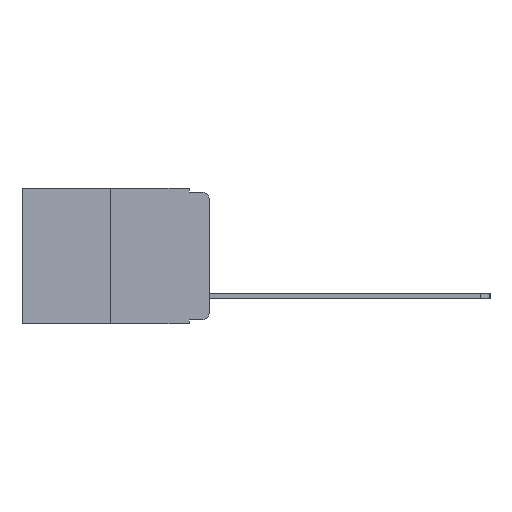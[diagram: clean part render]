
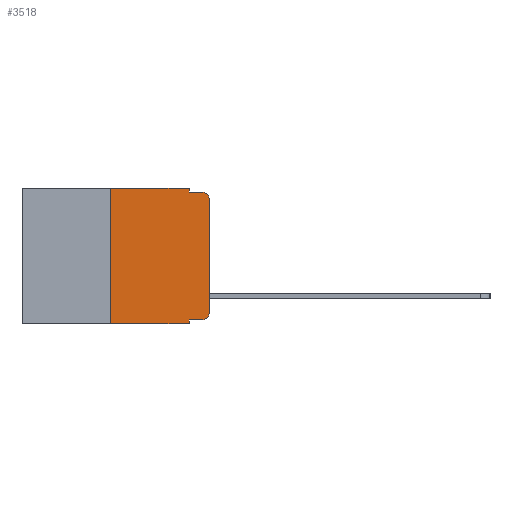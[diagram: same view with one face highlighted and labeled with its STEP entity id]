
A CAD part, left-side view. The second image highlights one B-rep face of the part: STEP entity #3518.
In plain terms, the highlighted planar face has unit normal (-1, 0, 0).
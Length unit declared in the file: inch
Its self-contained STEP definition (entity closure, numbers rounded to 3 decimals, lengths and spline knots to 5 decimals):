
#81 = CARTESIAN_POINT ( 'NONE',  ( 0., 0.473, 0. ) ) ;
#176 = ORIENTED_EDGE ( 'NONE', *, *, #246, .F. ) ;
#246 = EDGE_CURVE ( 'NONE', #16727, #5593, #1035, .T. ) ;
#524 = CARTESIAN_POINT ( 'NONE',  ( 0., 0.25, -0.343 ) ) ;
#882 = DIRECTION ( 'NONE',  ( 0., 0., -1. ) ) ;
#1035 = LINE ( 'NONE', #6684, #17609 ) ;
#1259 = ORIENTED_EDGE ( 'NONE', *, *, #16861, .T. ) ;
#1407 = EDGE_CURVE ( 'NONE', #2608, #8462, #6158, .T. ) ;
#1764 = DIRECTION ( 'NONE',  ( 0., 0., 1. ) ) ;
#1791 = ORIENTED_EDGE ( 'NONE', *, *, #15820, .T. ) ;
#1951 = CARTESIAN_POINT ( 'NONE',  ( 0., 0.02, -0.03 ) ) ;
#1986 = EDGE_CURVE ( 'NONE', #16727, #6013, #12176, .T. ) ;
#1997 = FACE_OUTER_BOUND ( 'NONE', #14314, .T. ) ;
#2320 = CARTESIAN_POINT ( 'NONE',  ( 0., 0.051, 0. ) ) ;
#2608 = VERTEX_POINT ( 'NONE', #2320 ) ;
#3518 = ADVANCED_FACE ( 'NONE', ( #1997 ), #7700, .F. ) ;
#3572 = ORIENTED_EDGE ( 'NONE', *, *, #1407, .F. ) ;
#3592 = DIRECTION ( 'NONE',  ( 0., 0., -1. ) ) ;
#4087 = ORIENTED_EDGE ( 'NONE', *, *, #7369, .F. ) ;
#4535 = DIRECTION ( 'NONE',  ( 1., 0., 0. ) ) ;
#4538 = CARTESIAN_POINT ( 'NONE',  ( 0., 0.051, -0.01 ) ) ;
#4600 = ORIENTED_EDGE ( 'NONE', *, *, #1986, .T. ) ;
#4641 = LINE ( 'NONE', #10688, #7469 ) ;
#4719 = EDGE_CURVE ( 'NONE', #8462, #19541, #13377, .T. ) ;
#4945 = VERTEX_POINT ( 'NONE', #5145 ) ;
#5006 = CARTESIAN_POINT ( 'NONE',  ( 0., 0., 0. ) ) ;
#5089 = DIRECTION ( 'NONE',  ( 0., 0., -1. ) ) ;
#5116 = CARTESIAN_POINT ( 'NONE',  ( 0., 0., -0.313 ) ) ;
#5145 = CARTESIAN_POINT ( 'NONE',  ( 0., 0., -0.03 ) ) ;
#5188 = CARTESIAN_POINT ( 'NONE',  ( 0., 0.25, 0. ) ) ;
#5298 = CARTESIAN_POINT ( 'NONE',  ( 0., 0.02, -0.01 ) ) ;
#5566 = VERTEX_POINT ( 'NONE', #5116 ) ;
#5593 = VERTEX_POINT ( 'NONE', #5188 ) ;
#5675 = CARTESIAN_POINT ( 'NONE',  ( 0., 0.051, -0.333 ) ) ;
#6013 = VERTEX_POINT ( 'NONE', #10946 ) ;
#6158 = LINE ( 'NONE', #6173, #18783 ) ;
#6173 = CARTESIAN_POINT ( 'NONE',  ( 0., 0.051, 0. ) ) ;
#6302 = CARTESIAN_POINT ( 'NONE',  ( 0., 0.02, -0.313 ) ) ;
#6607 = DIRECTION ( 'NONE',  ( 0., -1., 0. ) ) ;
#6684 = CARTESIAN_POINT ( 'NONE',  ( 0., 0.25, 0. ) ) ;
#6751 = LINE ( 'NONE', #81, #14245 ) ;
#6924 = EDGE_CURVE ( 'NONE', #4945, #19541, #13779, .T. ) ;
#7068 = DIRECTION ( 'NONE',  ( 0., 0., 1. ) ) ;
#7220 = ORIENTED_EDGE ( 'NONE', *, *, #6924, .T. ) ;
#7369 = EDGE_CURVE ( 'NONE', #5593, #2608, #6751, .T. ) ;
#7469 = VECTOR ( 'NONE', #12314, 39.37008 ) ;
#7700 = PLANE ( 'NONE',  #14649 ) ;
#7898 = AXIS2_PLACEMENT_3D ( 'NONE', #6302, #17373, #7928 ) ;
#7928 = DIRECTION ( 'NONE',  ( 0., 0., -1. ) ) ;
#8009 = EDGE_CURVE ( 'NONE', #5566, #4945, #9740, .T. ) ;
#8211 = LINE ( 'NONE', #14685, #16122 ) ;
#8462 = VERTEX_POINT ( 'NONE', #4538 ) ;
#9450 = ORIENTED_EDGE ( 'NONE', *, *, #19978, .F. ) ;
#9488 = CARTESIAN_POINT ( 'NONE',  ( 0., 0.051, -0.01 ) ) ;
#9740 = LINE ( 'NONE', #5006, #18084 ) ;
#10688 = CARTESIAN_POINT ( 'NONE',  ( 0., 0.051, -0.333 ) ) ;
#10946 = CARTESIAN_POINT ( 'NONE',  ( 0., 0.051, -0.343 ) ) ;
#11274 = VERTEX_POINT ( 'NONE', #5675 ) ;
#12176 = LINE ( 'NONE', #20471, #16317 ) ;
#12314 = DIRECTION ( 'NONE',  ( 0., -1., 0. ) ) ;
#12633 = VERTEX_POINT ( 'NONE', #19399 ) ;
#13283 = DIRECTION ( 'NONE',  ( -1., 0., 0. ) ) ;
#13377 = LINE ( 'NONE', #9488, #16532 ) ;
#13779 = CIRCLE ( 'NONE', #19758, 0.02 ) ;
#14180 = CARTESIAN_POINT ( 'NONE',  ( 0., 0.473, 0. ) ) ;
#14245 = VECTOR ( 'NONE', #6607, 39.37008 ) ;
#14314 = EDGE_LOOP ( 'NONE', ( #19293, #7220, #19980, #3572, #4087, #176, #4600, #9450, #1259, #1791 ) ) ;
#14649 = AXIS2_PLACEMENT_3D ( 'NONE', #14180, #4535, #15730 ) ;
#14685 = CARTESIAN_POINT ( 'NONE',  ( 0., 0.051, 0. ) ) ;
#15730 = DIRECTION ( 'NONE',  ( 0., 0., -1. ) ) ;
#15820 = EDGE_CURVE ( 'NONE', #12633, #5566, #19831, .T. ) ;
#16122 = VECTOR ( 'NONE', #5089, 39.37008 ) ;
#16317 = VECTOR ( 'NONE', #20496, 39.37008 ) ;
#16532 = VECTOR ( 'NONE', #20440, 39.37008 ) ;
#16727 = VERTEX_POINT ( 'NONE', #524 ) ;
#16861 = EDGE_CURVE ( 'NONE', #11274, #12633, #4641, .T. ) ;
#17373 = DIRECTION ( 'NONE',  ( -1., 0., 0. ) ) ;
#17609 = VECTOR ( 'NONE', #7068, 39.37008 ) ;
#18084 = VECTOR ( 'NONE', #1764, 39.37008 ) ;
#18783 = VECTOR ( 'NONE', #882, 39.37008 ) ;
#19293 = ORIENTED_EDGE ( 'NONE', *, *, #8009, .T. ) ;
#19399 = CARTESIAN_POINT ( 'NONE',  ( 0., 0.02, -0.333 ) ) ;
#19541 = VERTEX_POINT ( 'NONE', #5298 ) ;
#19758 = AXIS2_PLACEMENT_3D ( 'NONE', #1951, #13283, #3592 ) ;
#19831 = CIRCLE ( 'NONE', #7898, 0.02 ) ;
#19978 = EDGE_CURVE ( 'NONE', #11274, #6013, #8211, .T. ) ;
#19980 = ORIENTED_EDGE ( 'NONE', *, *, #4719, .F. ) ;
#20440 = DIRECTION ( 'NONE',  ( 0., -1., 0. ) ) ;
#20471 = CARTESIAN_POINT ( 'NONE',  ( 0., 0.473, -0.343 ) ) ;
#20496 = DIRECTION ( 'NONE',  ( 0., -1., 0. ) ) ;
